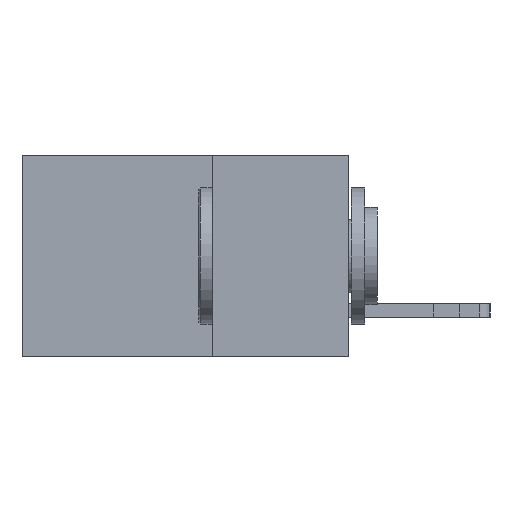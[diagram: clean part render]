
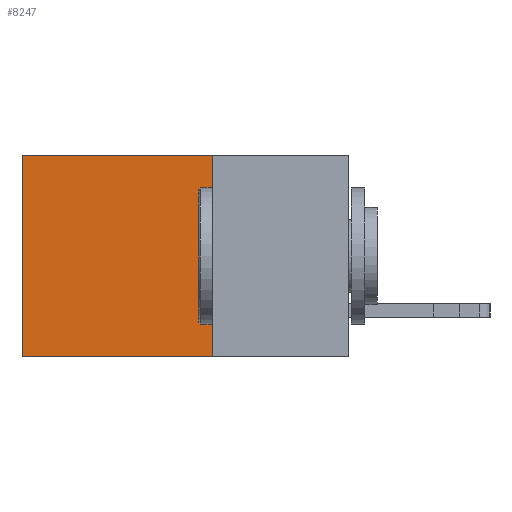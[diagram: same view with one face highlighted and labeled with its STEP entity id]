
A CAD part, left-side view. The second image highlights one B-rep face of the part: STEP entity #8247.
In plain terms, the highlighted planar face has unit normal (-1, 0, 0).
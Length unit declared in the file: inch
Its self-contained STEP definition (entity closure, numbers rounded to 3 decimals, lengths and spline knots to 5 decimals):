
#3 = VERTEX_POINT ( 'NONE', #2597 ) ;
#1914 = AXIS2_PLACEMENT_3D ( 'NONE', #9828, #9753, #9710 ) ;
#1950 = LINE ( 'NONE', #16775, #5647 ) ;
#2017 = VECTOR ( 'NONE', #17110, 39.37008 ) ;
#2116 = ORIENTED_EDGE ( 'NONE', *, *, #16033, .F. ) ;
#2597 = CARTESIAN_POINT ( 'NONE',  ( 0.2615, 0.25, 0. ) ) ;
#3306 = CARTESIAN_POINT ( 'NONE',  ( 0.2615, 0.6, 0. ) ) ;
#4662 = VERTEX_POINT ( 'NONE', #11606 ) ;
#5142 = DIRECTION ( 'NONE',  ( 0., 1., 0. ) ) ;
#5282 = VERTEX_POINT ( 'NONE', #3306 ) ;
#5639 = DIRECTION ( 'NONE',  ( 0., 1., 0. ) ) ;
#5647 = VECTOR ( 'NONE', #5639, 39.37008 ) ;
#7211 = EDGE_CURVE ( 'NONE', #3, #5282, #8383, .T. ) ;
#8247 = ADVANCED_FACE ( 'NONE', ( #8753 ), #9971, .F. ) ;
#8321 = ORIENTED_EDGE ( 'NONE', *, *, #13303, .T. ) ;
#8383 = LINE ( 'NONE', #14945, #15829 ) ;
#8738 = LINE ( 'NONE', #16087, #14838 ) ;
#8753 = FACE_OUTER_BOUND ( 'NONE', #10342, .T. ) ;
#9136 = DIRECTION ( 'NONE',  ( 0., 0., -1. ) ) ;
#9710 = DIRECTION ( 'NONE',  ( 0., 0., -1. ) ) ;
#9753 = DIRECTION ( 'NONE',  ( 1., 0., 0. ) ) ;
#9828 = CARTESIAN_POINT ( 'NONE',  ( 0.2615, 0.25, -0.37 ) ) ;
#9971 = PLANE ( 'NONE',  #1914 ) ;
#10342 = EDGE_LOOP ( 'NONE', ( #8321, #11747, #2116, #17402 ) ) ;
#10550 = CARTESIAN_POINT ( 'NONE',  ( 0.2615, 0.25, -0.37 ) ) ;
#11606 = CARTESIAN_POINT ( 'NONE',  ( 0.2615, 0.6, -0.37 ) ) ;
#11747 = ORIENTED_EDGE ( 'NONE', *, *, #15731, .F. ) ;
#13303 = EDGE_CURVE ( 'NONE', #5282, #4662, #16820, .T. ) ;
#14383 = CARTESIAN_POINT ( 'NONE',  ( 0.2615, 0.6, -0.37 ) ) ;
#14838 = VECTOR ( 'NONE', #9136, 39.37008 ) ;
#14945 = CARTESIAN_POINT ( 'NONE',  ( 0.2615, 0.25, 0. ) ) ;
#15731 = EDGE_CURVE ( 'NONE', #18010, #4662, #1950, .T. ) ;
#15829 = VECTOR ( 'NONE', #5142, 39.37008 ) ;
#16033 = EDGE_CURVE ( 'NONE', #3, #18010, #8738, .T. ) ;
#16087 = CARTESIAN_POINT ( 'NONE',  ( 0.2615, 0.25, -0.37 ) ) ;
#16775 = CARTESIAN_POINT ( 'NONE',  ( 0.2615, 0.25, -0.37 ) ) ;
#16820 = LINE ( 'NONE', #14383, #2017 ) ;
#17110 = DIRECTION ( 'NONE',  ( 0., 0., -1. ) ) ;
#17402 = ORIENTED_EDGE ( 'NONE', *, *, #7211, .T. ) ;
#18010 = VERTEX_POINT ( 'NONE', #10550 ) ;
